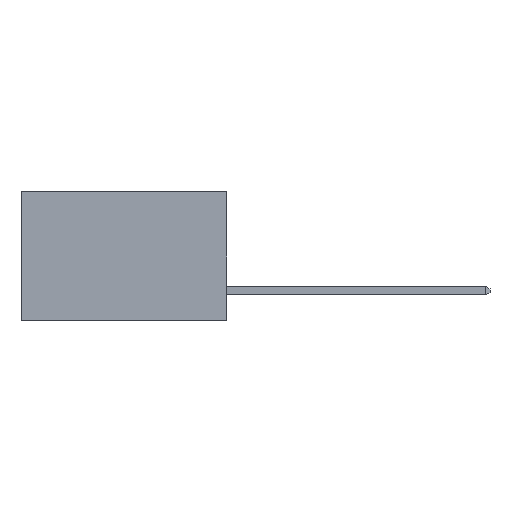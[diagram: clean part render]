
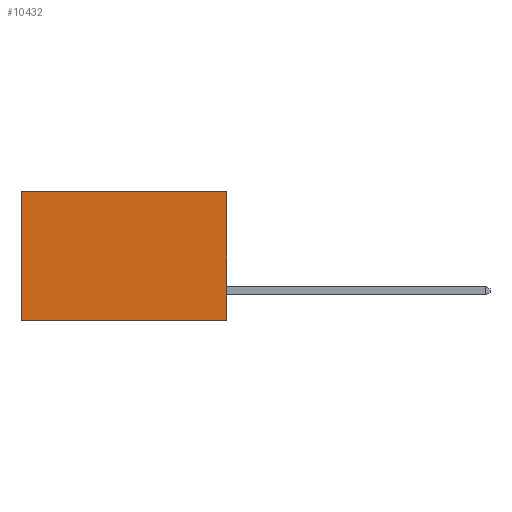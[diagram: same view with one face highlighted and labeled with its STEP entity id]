
A CAD part, left-side view. The second image highlights one B-rep face of the part: STEP entity #10432.
In plain terms, the highlighted planar face has unit normal (-1, 0, 0).
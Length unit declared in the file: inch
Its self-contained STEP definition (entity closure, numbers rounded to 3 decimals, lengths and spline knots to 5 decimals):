
#888 = DIRECTION ( 'NONE',  ( 0., 1., 0. ) ) ;
#1093 = LINE ( 'NONE', #1272, #6710 ) ;
#1272 = CARTESIAN_POINT ( 'NONE',  ( 0.277, 0., 0. ) ) ;
#1285 = VECTOR ( 'NONE', #5084, 39.37008 ) ;
#1752 = DIRECTION ( 'NONE',  ( 0., 0., -1. ) ) ;
#2069 = EDGE_LOOP ( 'NONE', ( #2469, #2391, #2209, #2199 ) ) ;
#2199 = ORIENTED_EDGE ( 'NONE', *, *, #2422, .T. ) ;
#2209 = ORIENTED_EDGE ( 'NONE', *, *, #2446, .F. ) ;
#2301 = EDGE_CURVE ( 'NONE', #6891, #8252, #10722, .T. ) ;
#2391 = ORIENTED_EDGE ( 'NONE', *, *, #2301, .F. ) ;
#2422 = EDGE_CURVE ( 'NONE', #6936, #3354, #1093, .T. ) ;
#2446 = EDGE_CURVE ( 'NONE', #6936, #6891, #10601, .T. ) ;
#2469 = ORIENTED_EDGE ( 'NONE', *, *, #4096, .T. ) ;
#2866 = DIRECTION ( 'NONE',  ( 1., 0., 0. ) ) ;
#3336 = CARTESIAN_POINT ( 'NONE',  ( 0.277, 0.59, 0. ) ) ;
#3354 = VERTEX_POINT ( 'NONE', #3336 ) ;
#3920 = CARTESIAN_POINT ( 'NONE',  ( 0.277, 0., -0.37 ) ) ;
#3966 = VECTOR ( 'NONE', #1752, 39.37008 ) ;
#4096 = EDGE_CURVE ( 'NONE', #3354, #8252, #10889, .T. ) ;
#4279 = FACE_OUTER_BOUND ( 'NONE', #2069, .T. ) ;
#4895 = CARTESIAN_POINT ( 'NONE',  ( 0.277, 0., -0.37 ) ) ;
#5084 = DIRECTION ( 'NONE',  ( 0., 1., 0. ) ) ;
#6515 = CARTESIAN_POINT ( 'NONE',  ( 0.277, 0., -0.37 ) ) ;
#6710 = VECTOR ( 'NONE', #888, 39.37008 ) ;
#6891 = VERTEX_POINT ( 'NONE', #3920 ) ;
#6936 = VERTEX_POINT ( 'NONE', #10854 ) ;
#8252 = VERTEX_POINT ( 'NONE', #9410 ) ;
#8458 = VECTOR ( 'NONE', #10152, 39.37008 ) ;
#9141 = DIRECTION ( 'NONE',  ( 0., 0., -1. ) ) ;
#9410 = CARTESIAN_POINT ( 'NONE',  ( 0.277, 0.59, -0.37 ) ) ;
#9909 = AXIS2_PLACEMENT_3D ( 'NONE', #4895, #2866, #9141 ) ;
#10152 = DIRECTION ( 'NONE',  ( 0., 0., -1. ) ) ;
#10168 = CARTESIAN_POINT ( 'NONE',  ( 0.277, 0.59, -0.37 ) ) ;
#10432 = ADVANCED_FACE ( 'NONE', ( #4279 ), #10772, .F. ) ;
#10601 = LINE ( 'NONE', #11723, #3966 ) ;
#10722 = LINE ( 'NONE', #6515, #1285 ) ;
#10772 = PLANE ( 'NONE',  #9909 ) ;
#10854 = CARTESIAN_POINT ( 'NONE',  ( 0.277, 0., 0. ) ) ;
#10889 = LINE ( 'NONE', #10168, #8458 ) ;
#11723 = CARTESIAN_POINT ( 'NONE',  ( 0.277, 0., -0.37 ) ) ;
